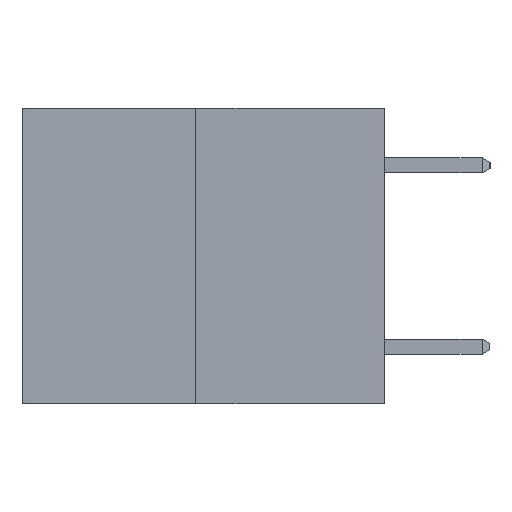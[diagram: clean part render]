
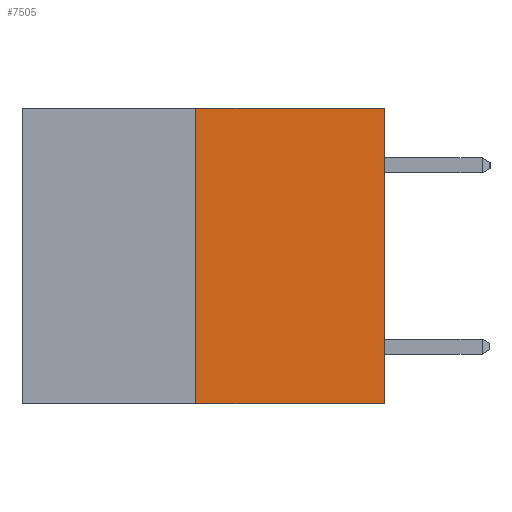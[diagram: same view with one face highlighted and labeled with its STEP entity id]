
A CAD part, left-side view. The second image highlights one B-rep face of the part: STEP entity #7505.
In plain terms, the highlighted planar face has unit normal (-1, 0, 0).
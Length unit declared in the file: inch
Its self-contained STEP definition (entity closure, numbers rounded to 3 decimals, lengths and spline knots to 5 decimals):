
#253 = CARTESIAN_POINT ( 'NONE',  ( 0., 0., 0. ) ) ;
#309 = EDGE_CURVE ( 'NONE', #8265, #8809, #7640, .T. ) ;
#1125 = CARTESIAN_POINT ( 'NONE',  ( 0., 0.6, 0. ) ) ;
#1162 = CARTESIAN_POINT ( 'NONE',  ( 0., 0.312, -0.49 ) ) ;
#1230 = PLANE ( 'NONE',  #2683 ) ;
#1295 = VECTOR ( 'NONE', #4826, 39.37008 ) ;
#1876 = CARTESIAN_POINT ( 'NONE',  ( 0., 0.312, 0. ) ) ;
#1895 = VECTOR ( 'NONE', #6757, 39.37008 ) ;
#1958 = CARTESIAN_POINT ( 'NONE',  ( 0., 0.6, 0. ) ) ;
#2143 = LINE ( 'NONE', #9166, #8488 ) ;
#2276 = EDGE_LOOP ( 'NONE', ( #2682, #3367, #5725, #9728 ) ) ;
#2352 = VERTEX_POINT ( 'NONE', #3120 ) ;
#2682 = ORIENTED_EDGE ( 'NONE', *, *, #9526, .F. ) ;
#2683 = AXIS2_PLACEMENT_3D ( 'NONE', #1958, #3404, #7924 ) ;
#2972 = CARTESIAN_POINT ( 'NONE',  ( 0., 0.6, -0.49 ) ) ;
#3067 = LINE ( 'NONE', #2972, #1895 ) ;
#3120 = CARTESIAN_POINT ( 'NONE',  ( 0., 0., -0.49 ) ) ;
#3367 = ORIENTED_EDGE ( 'NONE', *, *, #8086, .T. ) ;
#3404 = DIRECTION ( 'NONE',  ( 1., 0., 0. ) ) ;
#4387 = VERTEX_POINT ( 'NONE', #1162 ) ;
#4826 = DIRECTION ( 'NONE',  ( 0., 0., 1. ) ) ;
#4890 = DIRECTION ( 'NONE',  ( 0., -1., 0. ) ) ;
#5443 = DIRECTION ( 'NONE',  ( 0., 0., 1. ) ) ;
#5725 = ORIENTED_EDGE ( 'NONE', *, *, #8295, .T. ) ;
#6608 = FACE_OUTER_BOUND ( 'NONE', #2276, .T. ) ;
#6757 = DIRECTION ( 'NONE',  ( 0., -1., 0. ) ) ;
#7505 = ADVANCED_FACE ( 'NONE', ( #6608 ), #1230, .F. ) ;
#7640 = LINE ( 'NONE', #1125, #7891 ) ;
#7891 = VECTOR ( 'NONE', #4890, 39.37008 ) ;
#7924 = DIRECTION ( 'NONE',  ( 0., 0., -1. ) ) ;
#8017 = LINE ( 'NONE', #9303, #1295 ) ;
#8086 = EDGE_CURVE ( 'NONE', #4387, #2352, #3067, .T. ) ;
#8265 = VERTEX_POINT ( 'NONE', #1876 ) ;
#8295 = EDGE_CURVE ( 'NONE', #2352, #8809, #8017, .T. ) ;
#8488 = VECTOR ( 'NONE', #5443, 39.37008 ) ;
#8809 = VERTEX_POINT ( 'NONE', #253 ) ;
#9166 = CARTESIAN_POINT ( 'NONE',  ( 0., 0.312, -0.49 ) ) ;
#9303 = CARTESIAN_POINT ( 'NONE',  ( 0., 0., 0. ) ) ;
#9526 = EDGE_CURVE ( 'NONE', #4387, #8265, #2143, .T. ) ;
#9728 = ORIENTED_EDGE ( 'NONE', *, *, #309, .F. ) ;
